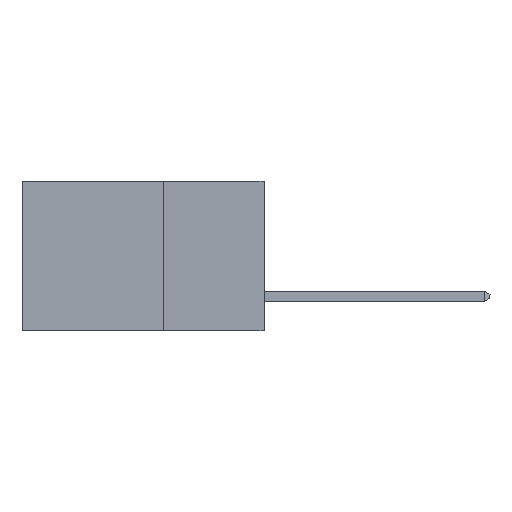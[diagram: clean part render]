
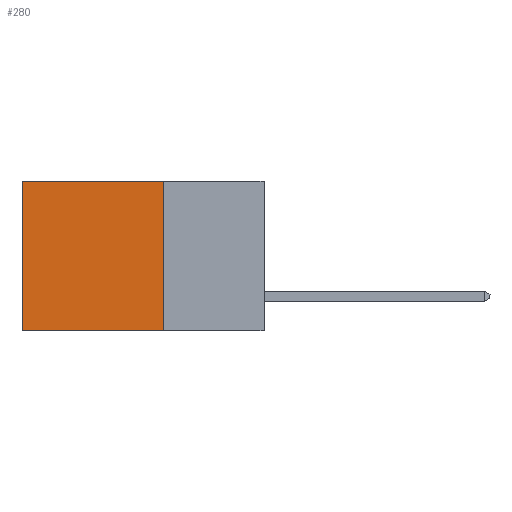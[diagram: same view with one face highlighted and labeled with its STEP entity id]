
A CAD part, left-side view. The second image highlights one B-rep face of the part: STEP entity #280.
In plain terms, the highlighted planar face has unit normal (-1, 0, 0).
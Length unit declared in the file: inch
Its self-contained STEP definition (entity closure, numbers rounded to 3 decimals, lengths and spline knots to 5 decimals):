
#19 = CARTESIAN_POINT ( 'NONE',  ( 0.2615, 0.25, -0.37 ) ) ;
#115 = DIRECTION ( 'NONE',  ( 0., 0., -1. ) ) ;
#116 = PLANE ( 'NONE',  #4565 ) ;
#157 = CARTESIAN_POINT ( 'NONE',  ( 0.2615, 0.25, -0.37 ) ) ;
#280 = ADVANCED_FACE ( 'NONE', ( #5758 ), #116, .F. ) ;
#2073 = VERTEX_POINT ( 'NONE', #3915 ) ;
#2202 = DIRECTION ( 'NONE',  ( 0., 0., -1. ) ) ;
#2438 = VECTOR ( 'NONE', #2467, 39.37008 ) ;
#2467 = DIRECTION ( 'NONE',  ( 0., 0., -1. ) ) ;
#2491 = LINE ( 'NONE', #5357, #8445 ) ;
#2630 = EDGE_CURVE ( 'NONE', #8290, #8497, #2491, .T. ) ;
#2910 = EDGE_LOOP ( 'NONE', ( #8452, #5538, #5499, #8582 ) ) ;
#3037 = DIRECTION ( 'NONE',  ( 0., 1., 0. ) ) ;
#3089 = LINE ( 'NONE', #5109, #8504 ) ;
#3499 = EDGE_CURVE ( 'NONE', #8497, #2073, #3833, .T. ) ;
#3833 = LINE ( 'NONE', #6025, #2438 ) ;
#3915 = CARTESIAN_POINT ( 'NONE',  ( 0.2615, 0.6, -0.37 ) ) ;
#4565 = AXIS2_PLACEMENT_3D ( 'NONE', #19, #8648, #2202 ) ;
#4643 = DIRECTION ( 'NONE',  ( 0., 1., 0. ) ) ;
#5109 = CARTESIAN_POINT ( 'NONE',  ( 0.2615, 0.25, -0.37 ) ) ;
#5357 = CARTESIAN_POINT ( 'NONE',  ( 0.2615, 0.25, 0. ) ) ;
#5499 = ORIENTED_EDGE ( 'NONE', *, *, #6595, .F. ) ;
#5538 = ORIENTED_EDGE ( 'NONE', *, *, #7345, .F. ) ;
#5758 = FACE_OUTER_BOUND ( 'NONE', #2910, .T. ) ;
#6025 = CARTESIAN_POINT ( 'NONE',  ( 0.2615, 0.6, -0.37 ) ) ;
#6120 = CARTESIAN_POINT ( 'NONE',  ( 0.2615, 0.25, -0.37 ) ) ;
#6475 = CARTESIAN_POINT ( 'NONE',  ( 0.2615, 0.6, 0. ) ) ;
#6547 = LINE ( 'NONE', #157, #8488 ) ;
#6595 = EDGE_CURVE ( 'NONE', #8290, #6712, #6547, .T. ) ;
#6712 = VERTEX_POINT ( 'NONE', #6120 ) ;
#7345 = EDGE_CURVE ( 'NONE', #6712, #2073, #3089, .T. ) ;
#8290 = VERTEX_POINT ( 'NONE', #8864 ) ;
#8445 = VECTOR ( 'NONE', #4643, 39.37008 ) ;
#8452 = ORIENTED_EDGE ( 'NONE', *, *, #3499, .T. ) ;
#8488 = VECTOR ( 'NONE', #115, 39.37008 ) ;
#8497 = VERTEX_POINT ( 'NONE', #6475 ) ;
#8504 = VECTOR ( 'NONE', #3037, 39.37008 ) ;
#8582 = ORIENTED_EDGE ( 'NONE', *, *, #2630, .T. ) ;
#8648 = DIRECTION ( 'NONE',  ( 1., 0., 0. ) ) ;
#8864 = CARTESIAN_POINT ( 'NONE',  ( 0.2615, 0.25, 0. ) ) ;
